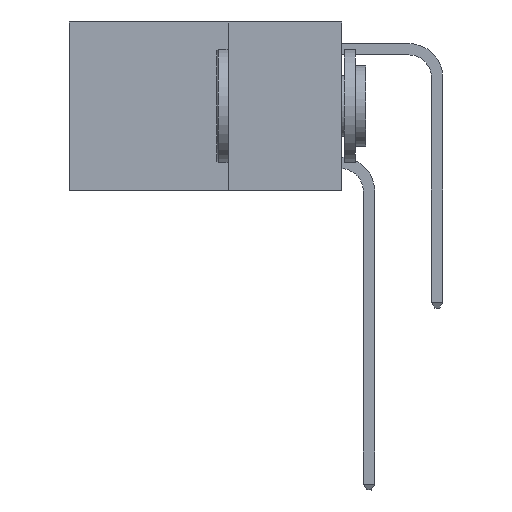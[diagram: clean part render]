
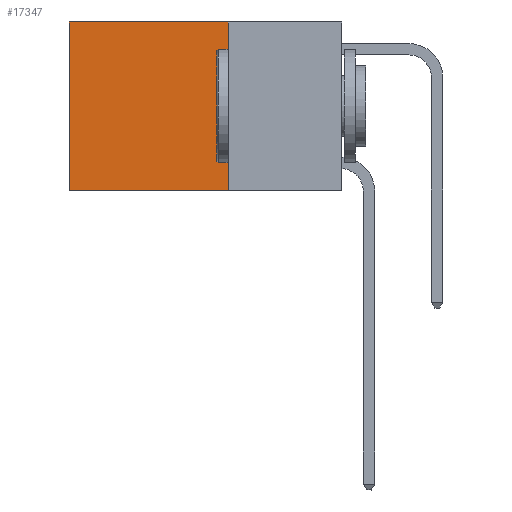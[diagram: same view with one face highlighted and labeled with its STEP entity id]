
A CAD part, left-side view. The second image highlights one B-rep face of the part: STEP entity #17347.
In plain terms, the highlighted planar face has unit normal (-1, 0, 0).
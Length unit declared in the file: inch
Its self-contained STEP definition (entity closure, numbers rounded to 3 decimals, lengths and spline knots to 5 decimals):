
#858 = CARTESIAN_POINT ( 'NONE',  ( 0.2625, 0.25, 0. ) ) ;
#960 = ORIENTED_EDGE ( 'NONE', *, *, #25327, .F. ) ;
#1470 = DIRECTION ( 'NONE',  ( 0., 0., -1. ) ) ;
#1582 = CARTESIAN_POINT ( 'NONE',  ( 0.2625, 0.25, 0. ) ) ;
#2961 = VECTOR ( 'NONE', #1470, 39.37008 ) ;
#4349 = VECTOR ( 'NONE', #21495, 39.37008 ) ;
#4994 = ORIENTED_EDGE ( 'NONE', *, *, #26524, .T. ) ;
#5105 = VERTEX_POINT ( 'NONE', #18933 ) ;
#5308 = AXIS2_PLACEMENT_3D ( 'NONE', #1582, #20179, #7781 ) ;
#5593 = CARTESIAN_POINT ( 'NONE',  ( 0.2625, 0.25, 0. ) ) ;
#5786 = CARTESIAN_POINT ( 'NONE',  ( 0.2625, 0.6, -0.37 ) ) ;
#7778 = CARTESIAN_POINT ( 'NONE',  ( 0.2625, 0.25, 0. ) ) ;
#7781 = DIRECTION ( 'NONE',  ( 0., 0., -1. ) ) ;
#7932 = DIRECTION ( 'NONE',  ( 0., 1., 0. ) ) ;
#8255 = VERTEX_POINT ( 'NONE', #5786 ) ;
#9787 = PLANE ( 'NONE',  #5308 ) ;
#10617 = CARTESIAN_POINT ( 'NONE',  ( 0.2625, 0.25, -0.37 ) ) ;
#11262 = DIRECTION ( 'NONE',  ( 0., 0., -1. ) ) ;
#12302 = EDGE_LOOP ( 'NONE', ( #4994, #19026, #960, #21994 ) ) ;
#14201 = LINE ( 'NONE', #21572, #19057 ) ;
#14264 = VERTEX_POINT ( 'NONE', #7778 ) ;
#14495 = VERTEX_POINT ( 'NONE', #10617 ) ;
#14580 = LINE ( 'NONE', #5593, #2961 ) ;
#15973 = LINE ( 'NONE', #858, #4349 ) ;
#15990 = EDGE_CURVE ( 'NONE', #14495, #8255, #16570, .T. ) ;
#16570 = LINE ( 'NONE', #24479, #21438 ) ;
#17011 = FACE_OUTER_BOUND ( 'NONE', #12302, .T. ) ;
#17347 = ADVANCED_FACE ( 'NONE', ( #17011 ), #9787, .F. ) ;
#18933 = CARTESIAN_POINT ( 'NONE',  ( 0.2625, 0.6, 0. ) ) ;
#19026 = ORIENTED_EDGE ( 'NONE', *, *, #15990, .F. ) ;
#19057 = VECTOR ( 'NONE', #11262, 39.37008 ) ;
#19347 = EDGE_CURVE ( 'NONE', #14264, #5105, #15973, .T. ) ;
#20179 = DIRECTION ( 'NONE',  ( 1., 0., 0. ) ) ;
#21438 = VECTOR ( 'NONE', #7932, 39.37008 ) ;
#21495 = DIRECTION ( 'NONE',  ( 0., 1., 0. ) ) ;
#21572 = CARTESIAN_POINT ( 'NONE',  ( 0.2625, 0.6, 0. ) ) ;
#21994 = ORIENTED_EDGE ( 'NONE', *, *, #19347, .T. ) ;
#24479 = CARTESIAN_POINT ( 'NONE',  ( 0.2625, 0.25, -0.37 ) ) ;
#25327 = EDGE_CURVE ( 'NONE', #14264, #14495, #14580, .T. ) ;
#26524 = EDGE_CURVE ( 'NONE', #5105, #8255, #14201, .T. ) ;
